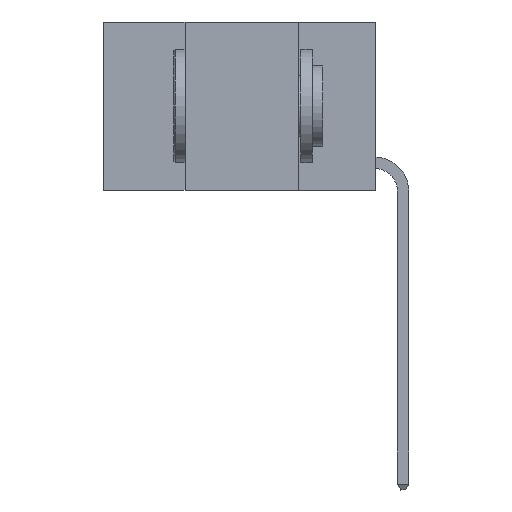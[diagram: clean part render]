
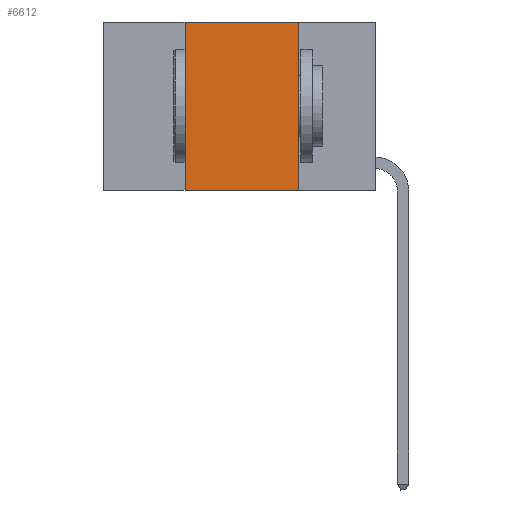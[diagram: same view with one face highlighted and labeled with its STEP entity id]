
A CAD part, left-side view. The second image highlights one B-rep face of the part: STEP entity #6612.
In plain terms, the highlighted planar face has unit normal (-1, 0, 0).
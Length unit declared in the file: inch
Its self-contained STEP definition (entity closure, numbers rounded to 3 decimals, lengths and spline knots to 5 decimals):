
#253 = VECTOR ( 'NONE', #21476, 39.37008 ) ;
#568 = DIRECTION ( 'NONE',  ( 0., 0., -1. ) ) ;
#810 = EDGE_CURVE ( 'NONE', #22171, #13739, #8181, .T. ) ;
#818 = DIRECTION ( 'NONE',  ( 0., 0., -1. ) ) ;
#2826 = VERTEX_POINT ( 'NONE', #17597 ) ;
#3855 = VERTEX_POINT ( 'NONE', #22007 ) ;
#6608 = EDGE_LOOP ( 'NONE', ( #23618, #16745, #8264, #22918 ) ) ;
#6612 = ADVANCED_FACE ( 'NONE', ( #11525 ), #19335, .F. ) ;
#7551 = DIRECTION ( 'NONE',  ( 0., -1., 0. ) ) ;
#7675 = EDGE_CURVE ( 'NONE', #3855, #13739, #24880, .T. ) ;
#8181 = LINE ( 'NONE', #8444, #10334 ) ;
#8264 = ORIENTED_EDGE ( 'NONE', *, *, #14113, .F. ) ;
#8444 = CARTESIAN_POINT ( 'NONE',  ( 0., 0.17, 0. ) ) ;
#10334 = VECTOR ( 'NONE', #568, 39.37008 ) ;
#10879 = CARTESIAN_POINT ( 'NONE',  ( 0., 0.42, 0. ) ) ;
#11525 = FACE_OUTER_BOUND ( 'NONE', #6608, .T. ) ;
#12570 = AXIS2_PLACEMENT_3D ( 'NONE', #15476, #14195, #818 ) ;
#13717 = CARTESIAN_POINT ( 'NONE',  ( 0., 0.17, -0.37 ) ) ;
#13739 = VERTEX_POINT ( 'NONE', #13717 ) ;
#13892 = VECTOR ( 'NONE', #7551, 39.37008 ) ;
#14113 = EDGE_CURVE ( 'NONE', #3855, #2826, #14714, .T. ) ;
#14195 = DIRECTION ( 'NONE',  ( 1., 0., 0. ) ) ;
#14390 = CARTESIAN_POINT ( 'NONE',  ( 0., 0.17, 0. ) ) ;
#14714 = LINE ( 'NONE', #10879, #22442 ) ;
#15476 = CARTESIAN_POINT ( 'NONE',  ( 0., 0.6, 0. ) ) ;
#15672 = CARTESIAN_POINT ( 'NONE',  ( 0., 0.6, 0. ) ) ;
#16149 = EDGE_CURVE ( 'NONE', #2826, #22171, #17599, .T. ) ;
#16745 = ORIENTED_EDGE ( 'NONE', *, *, #16149, .F. ) ;
#17597 = CARTESIAN_POINT ( 'NONE',  ( 0., 0.42, 0. ) ) ;
#17599 = LINE ( 'NONE', #15672, #253 ) ;
#19335 = PLANE ( 'NONE',  #12570 ) ;
#21476 = DIRECTION ( 'NONE',  ( 0., -1., 0. ) ) ;
#22007 = CARTESIAN_POINT ( 'NONE',  ( 0., 0.42, -0.37 ) ) ;
#22171 = VERTEX_POINT ( 'NONE', #14390 ) ;
#22342 = DIRECTION ( 'NONE',  ( 0., 0., 1. ) ) ;
#22442 = VECTOR ( 'NONE', #22342, 39.37008 ) ;
#22918 = ORIENTED_EDGE ( 'NONE', *, *, #7675, .T. ) ;
#23094 = CARTESIAN_POINT ( 'NONE',  ( 0., 0.6, -0.37 ) ) ;
#23618 = ORIENTED_EDGE ( 'NONE', *, *, #810, .F. ) ;
#24880 = LINE ( 'NONE', #23094, #13892 ) ;
